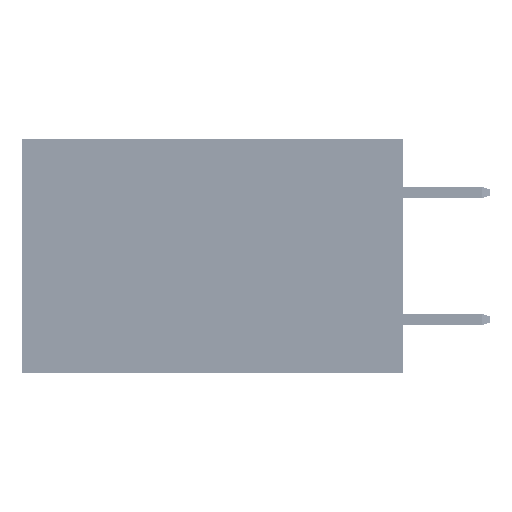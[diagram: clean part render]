
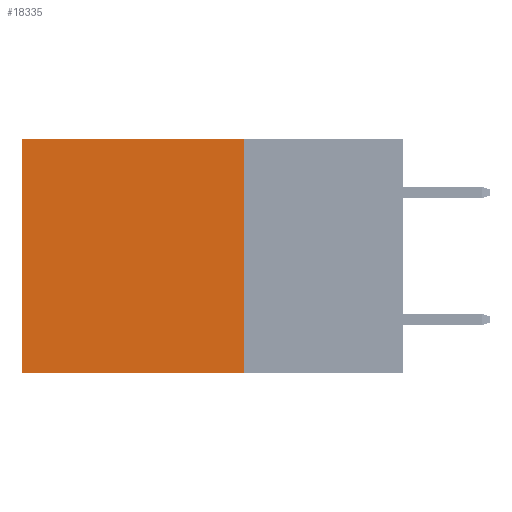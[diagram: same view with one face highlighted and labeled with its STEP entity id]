
A CAD part, left-side view. The second image highlights one B-rep face of the part: STEP entity #18335.
In plain terms, the highlighted planar face has unit normal (-1, 0, 0).
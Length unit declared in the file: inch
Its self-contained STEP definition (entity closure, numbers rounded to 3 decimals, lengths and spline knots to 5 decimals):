
#854 = CARTESIAN_POINT ( 'NONE',  ( 0.2875, 0.25, 0. ) ) ;
#1559 = CARTESIAN_POINT ( 'NONE',  ( 0.2875, 0.25, 0. ) ) ;
#1884 = LINE ( 'NONE', #41092, #32710 ) ;
#3325 = EDGE_LOOP ( 'NONE', ( #34193, #13848, #25663, #32015 ) ) ;
#8076 = VECTOR ( 'NONE', #24177, 39.37008 ) ;
#10467 = EDGE_CURVE ( 'NONE', #32772, #11383, #1884, .T. ) ;
#11182 = FACE_OUTER_BOUND ( 'NONE', #3325, .T. ) ;
#11383 = VERTEX_POINT ( 'NONE', #37031 ) ;
#11584 = DIRECTION ( 'NONE',  ( 0., 0., -1. ) ) ;
#13848 = ORIENTED_EDGE ( 'NONE', *, *, #10467, .F. ) ;
#15706 = VECTOR ( 'NONE', #11584, 39.37008 ) ;
#17207 = DIRECTION ( 'NONE',  ( 0., 0., -1. ) ) ;
#18335 = ADVANCED_FACE ( 'NONE', ( #11182 ), #19598, .F. ) ;
#19175 = AXIS2_PLACEMENT_3D ( 'NONE', #41942, #22944, #35234 ) ;
#19598 = PLANE ( 'NONE',  #19175 ) ;
#22944 = DIRECTION ( 'NONE',  ( 1., 0., 0. ) ) ;
#24177 = DIRECTION ( 'NONE',  ( 0., 1., 0. ) ) ;
#25663 = ORIENTED_EDGE ( 'NONE', *, *, #28431, .F. ) ;
#27188 = CARTESIAN_POINT ( 'NONE',  ( 0.2875, 0.6, 0. ) ) ;
#27350 = VERTEX_POINT ( 'NONE', #35109 ) ;
#28431 = EDGE_CURVE ( 'NONE', #27350, #32772, #36676, .T. ) ;
#29690 = VECTOR ( 'NONE', #17207, 39.37008 ) ;
#32015 = ORIENTED_EDGE ( 'NONE', *, *, #38768, .T. ) ;
#32710 = VECTOR ( 'NONE', #33399, 39.37008 ) ;
#32772 = VERTEX_POINT ( 'NONE', #33775 ) ;
#33399 = DIRECTION ( 'NONE',  ( 0., 1., 0. ) ) ;
#33775 = CARTESIAN_POINT ( 'NONE',  ( 0.2875, 0.25, -0.37 ) ) ;
#34193 = ORIENTED_EDGE ( 'NONE', *, *, #42101, .T. ) ;
#35109 = CARTESIAN_POINT ( 'NONE',  ( 0.2875, 0.25, 0. ) ) ;
#35234 = DIRECTION ( 'NONE',  ( 0., 0., -1. ) ) ;
#36676 = LINE ( 'NONE', #1559, #29690 ) ;
#37031 = CARTESIAN_POINT ( 'NONE',  ( 0.2875, 0.6, -0.37 ) ) ;
#37621 = VERTEX_POINT ( 'NONE', #44907 ) ;
#38768 = EDGE_CURVE ( 'NONE', #27350, #37621, #39294, .T. ) ;
#39294 = LINE ( 'NONE', #854, #8076 ) ;
#41092 = CARTESIAN_POINT ( 'NONE',  ( 0.2875, 0.25, -0.37 ) ) ;
#41942 = CARTESIAN_POINT ( 'NONE',  ( 0.2875, 0.25, 0. ) ) ;
#42082 = LINE ( 'NONE', #27188, #15706 ) ;
#42101 = EDGE_CURVE ( 'NONE', #37621, #11383, #42082, .T. ) ;
#44907 = CARTESIAN_POINT ( 'NONE',  ( 0.2875, 0.6, 0. ) ) ;
